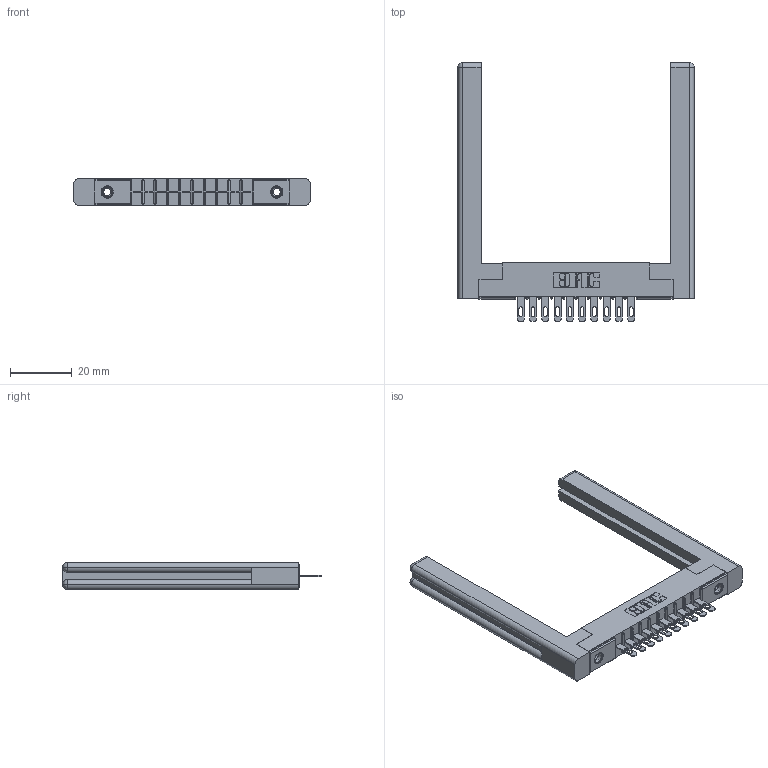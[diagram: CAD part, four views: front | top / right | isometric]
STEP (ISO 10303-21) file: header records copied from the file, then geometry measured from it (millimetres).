
FILE_DESCRIPTION (( 'STEP AP203' ), '1' );
FILE_NAME ('306-010-500-158.STEP', '2019-09-11T19:15:57', ( '' ), ( '' ), 'SwSTEP 2.0', 'SolidWorks 2016', '' );
FILE_SCHEMA (( 'CONFIG_CONTROL_DESIGN' ));
Length unit declared in the file: inch
Products named in the file (5): 306-010-500-158; 307-220-058; 306-290-001_100; 306 Part_.156 Dia; 345-250-001_345-250-001-102
Assembly tree (15 placements, depth 2):
  306-010-500-158
    306 Part_.156 Dia
    306-290-001_100  x10
    345-250-001_345-250-001-102  x2
    307-220-058  x2
Bounding box: 76.25 x 83.52 x 8.71 mm (x, y, z)
Volume: 12836.2 mm3; surface area: 12754.8 mm2
Topology: 15 solids, 15 shells, 1018 faces, 2820 edges, 1812 vertices
Faces by surface type: plane 652, cylinder 302, sphere 40, cone 12, torus 12
Entity records: 16268 total; most frequent: CARTESIAN_POINT 2736, DIRECTION 2657, ORIENTED_EDGE 2650, EDGE_CURVE 1325, VECTOR 1011, LINE 1011, VERTEX_POINT 848, AXIS2_PLACEMENT_3D 823
